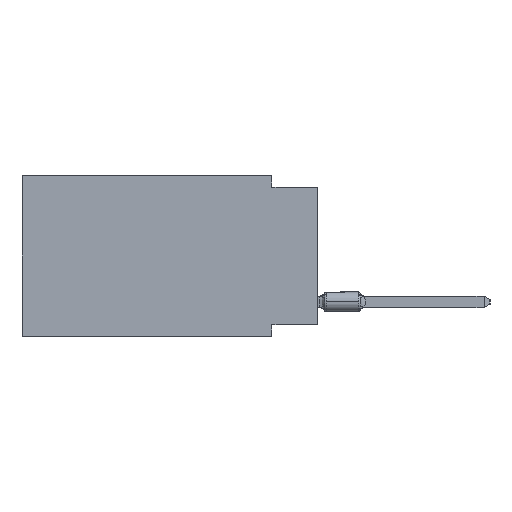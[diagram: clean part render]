
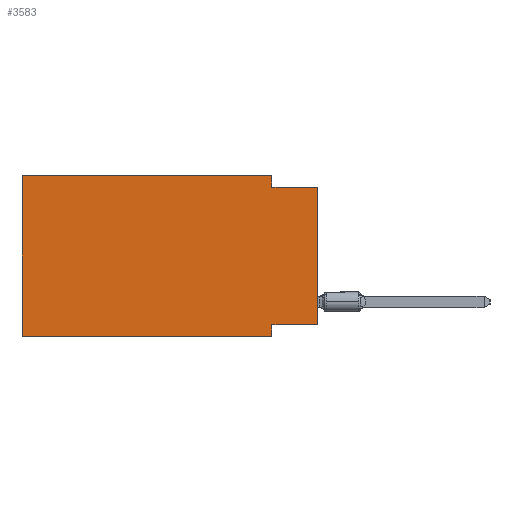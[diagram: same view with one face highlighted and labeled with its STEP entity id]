
A CAD part, left-side view. The second image highlights one B-rep face of the part: STEP entity #3583.
In plain terms, the highlighted planar face has unit normal (-1, 0, 0).
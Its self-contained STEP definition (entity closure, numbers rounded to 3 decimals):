
#331 = VECTOR ( 'NONE', #53597, 1000. ) ;
#801 = CARTESIAN_POINT ( 'NONE',  ( 0., 0., -0.635 ) ) ;
#1609 = LINE ( 'NONE', #48809, #50187 ) ;
#1931 = DIRECTION ( 'NONE',  ( 0., 0., -1. ) ) ;
#2736 = LINE ( 'NONE', #12668, #32970 ) ;
#3583 = ADVANCED_FACE ( 'NONE', ( #31309 ), #50241, .F. ) ;
#4095 = CARTESIAN_POINT ( 'NONE',  ( 0., 0., 0. ) ) ;
#5772 = CARTESIAN_POINT ( 'NONE',  ( 0., 0., -8.255 ) ) ;
#7643 = CARTESIAN_POINT ( 'NONE',  ( 0., 16.383, 0. ) ) ;
#9129 = EDGE_CURVE ( 'NONE', #30899, #56760, #45081, .T. ) ;
#10336 = DIRECTION ( 'NONE',  ( 0., 0., -1. ) ) ;
#10748 = VERTEX_POINT ( 'NONE', #7643 ) ;
#10759 = CARTESIAN_POINT ( 'NONE',  ( 0., 16.383, -8.89 ) ) ;
#11200 = EDGE_CURVE ( 'NONE', #10748, #40181, #18111, .T. ) ;
#11338 = DIRECTION ( 'NONE',  ( 0., -1., 0. ) ) ;
#12606 = EDGE_CURVE ( 'NONE', #16482, #56760, #24736, .T. ) ;
#12668 = CARTESIAN_POINT ( 'NONE',  ( 0., 16.383, 0. ) ) ;
#13468 = DIRECTION ( 'NONE',  ( 0., -1., 0. ) ) ;
#14429 = EDGE_CURVE ( 'NONE', #41657, #30899, #33343, .T. ) ;
#16482 = VERTEX_POINT ( 'NONE', #54001 ) ;
#18111 = LINE ( 'NONE', #51034, #43823 ) ;
#18637 = CARTESIAN_POINT ( 'NONE',  ( 0., 0., -0.635 ) ) ;
#20846 = EDGE_LOOP ( 'NONE', ( #24854, #44214, #60711, #41211, #47953, #29634, #25267, #45376 ) ) ;
#23207 = DIRECTION ( 'NONE',  ( 0., 0., -1. ) ) ;
#23529 = DIRECTION ( 'NONE',  ( 1., 0., 0. ) ) ;
#24736 = LINE ( 'NONE', #10759, #331 ) ;
#24854 = ORIENTED_EDGE ( 'NONE', *, *, #56079, .T. ) ;
#25267 = ORIENTED_EDGE ( 'NONE', *, *, #9129, .F. ) ;
#26549 = CARTESIAN_POINT ( 'NONE',  ( 0., 2.54, -8.89 ) ) ;
#26639 = CARTESIAN_POINT ( 'NONE',  ( 0., 16.383, 0. ) ) ;
#29634 = ORIENTED_EDGE ( 'NONE', *, *, #12606, .T. ) ;
#30177 = VECTOR ( 'NONE', #46335, 1000. ) ;
#30899 = VERTEX_POINT ( 'NONE', #35416 ) ;
#31309 = FACE_OUTER_BOUND ( 'NONE', #20846, .T. ) ;
#32407 = CARTESIAN_POINT ( 'NONE',  ( 0., 0., -8.255 ) ) ;
#32536 = DIRECTION ( 'NONE',  ( 0., 0., 1. ) ) ;
#32970 = VECTOR ( 'NONE', #32536, 1000. ) ;
#33343 = LINE ( 'NONE', #32407, #46960 ) ;
#34928 = LINE ( 'NONE', #801, #54714 ) ;
#35416 = CARTESIAN_POINT ( 'NONE',  ( 0., 2.54, -8.255 ) ) ;
#37367 = DIRECTION ( 'NONE',  ( 0., 1., 0. ) ) ;
#39557 = VECTOR ( 'NONE', #1931, 1000. ) ;
#40181 = VERTEX_POINT ( 'NONE', #45317 ) ;
#41211 = ORIENTED_EDGE ( 'NONE', *, *, #11200, .F. ) ;
#41657 = VERTEX_POINT ( 'NONE', #5772 ) ;
#43823 = VECTOR ( 'NONE', #13468, 1000. ) ;
#44214 = ORIENTED_EDGE ( 'NONE', *, *, #50768, .F. ) ;
#45081 = LINE ( 'NONE', #54111, #39557 ) ;
#45317 = CARTESIAN_POINT ( 'NONE',  ( 0., 2.54, 0. ) ) ;
#45376 = ORIENTED_EDGE ( 'NONE', *, *, #14429, .F. ) ;
#46335 = DIRECTION ( 'NONE',  ( 0., 0., 1. ) ) ;
#46960 = VECTOR ( 'NONE', #37367, 1000. ) ;
#47953 = ORIENTED_EDGE ( 'NONE', *, *, #53788, .F. ) ;
#48809 = CARTESIAN_POINT ( 'NONE',  ( 0., 2.54, 0. ) ) ;
#50187 = VECTOR ( 'NONE', #10336, 1000. ) ;
#50241 = PLANE ( 'NONE',  #61094 ) ;
#50768 = EDGE_CURVE ( 'NONE', #56398, #54663, #34928, .T. ) ;
#50832 = CARTESIAN_POINT ( 'NONE',  ( 0., 2.54, -0.635 ) ) ;
#51034 = CARTESIAN_POINT ( 'NONE',  ( 0., 16.383, 0. ) ) ;
#53597 = DIRECTION ( 'NONE',  ( 0., -1., 0. ) ) ;
#53788 = EDGE_CURVE ( 'NONE', #16482, #10748, #2736, .T. ) ;
#54001 = CARTESIAN_POINT ( 'NONE',  ( 0., 16.383, -8.89 ) ) ;
#54111 = CARTESIAN_POINT ( 'NONE',  ( 0., 2.54, -8.89 ) ) ;
#54663 = VERTEX_POINT ( 'NONE', #18637 ) ;
#54714 = VECTOR ( 'NONE', #11338, 1000. ) ;
#54718 = LINE ( 'NONE', #4095, #30177 ) ;
#56079 = EDGE_CURVE ( 'NONE', #41657, #54663, #54718, .T. ) ;
#56398 = VERTEX_POINT ( 'NONE', #50832 ) ;
#56760 = VERTEX_POINT ( 'NONE', #26549 ) ;
#58182 = EDGE_CURVE ( 'NONE', #40181, #56398, #1609, .T. ) ;
#60711 = ORIENTED_EDGE ( 'NONE', *, *, #58182, .F. ) ;
#61094 = AXIS2_PLACEMENT_3D ( 'NONE', #26639, #23529, #23207 ) ;
